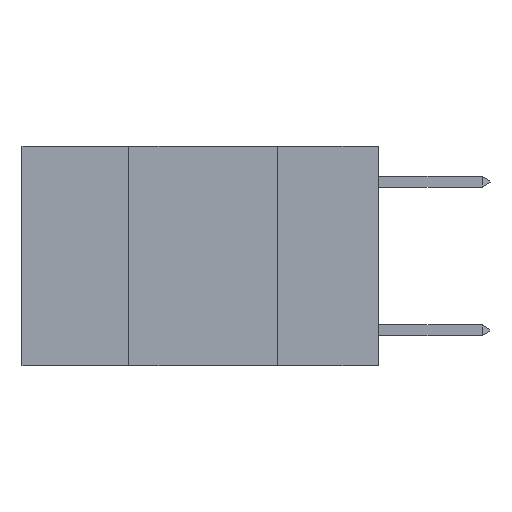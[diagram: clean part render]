
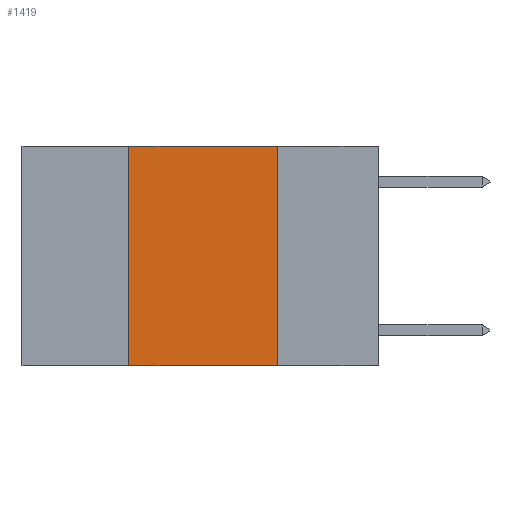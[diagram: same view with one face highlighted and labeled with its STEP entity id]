
A CAD part, left-side view. The second image highlights one B-rep face of the part: STEP entity #1419.
In plain terms, the highlighted planar face has unit normal (-1, 0, 0).
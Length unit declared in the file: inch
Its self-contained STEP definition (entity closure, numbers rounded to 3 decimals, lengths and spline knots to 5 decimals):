
#207 = CARTESIAN_POINT ( 'NONE',  ( 0., 0.17, 0. ) ) ;
#1419 = ADVANCED_FACE ( 'NONE', ( #8242 ), #20766, .F. ) ;
#2036 = VECTOR ( 'NONE', #12750, 39.37008 ) ;
#2325 = DIRECTION ( 'NONE',  ( 0., -1., 0. ) ) ;
#2397 = VERTEX_POINT ( 'NONE', #18102 ) ;
#2954 = LINE ( 'NONE', #10065, #5689 ) ;
#3046 = CARTESIAN_POINT ( 'NONE',  ( 0., 0.42, -0.37 ) ) ;
#3120 = LINE ( 'NONE', #10228, #6499 ) ;
#4056 = LINE ( 'NONE', #207, #2036 ) ;
#5689 = VECTOR ( 'NONE', #17118, 39.37008 ) ;
#6343 = VERTEX_POINT ( 'NONE', #3046 ) ;
#6477 = DIRECTION ( 'NONE',  ( 0., 0., -1. ) ) ;
#6499 = VECTOR ( 'NONE', #12293, 39.37008 ) ;
#6573 = ORIENTED_EDGE ( 'NONE', *, *, #15340, .F. ) ;
#7079 = ORIENTED_EDGE ( 'NONE', *, *, #15444, .F. ) ;
#8242 = FACE_OUTER_BOUND ( 'NONE', #8415, .T. ) ;
#8415 = EDGE_LOOP ( 'NONE', ( #7079, #14793, #6573, #14806 ) ) ;
#10065 = CARTESIAN_POINT ( 'NONE',  ( 0., 0.6, -0.37 ) ) ;
#10228 = CARTESIAN_POINT ( 'NONE',  ( 0., 0.42, 0. ) ) ;
#11942 = CARTESIAN_POINT ( 'NONE',  ( 0., 0.6, 0. ) ) ;
#12293 = DIRECTION ( 'NONE',  ( 0., 0., 1. ) ) ;
#12750 = DIRECTION ( 'NONE',  ( 0., 0., -1. ) ) ;
#14298 = LINE ( 'NONE', #18222, #17286 ) ;
#14793 = ORIENTED_EDGE ( 'NONE', *, *, #22801, .F. ) ;
#14806 = ORIENTED_EDGE ( 'NONE', *, *, #19401, .T. ) ;
#15340 = EDGE_CURVE ( 'NONE', #6343, #15740, #3120, .T. ) ;
#15444 = EDGE_CURVE ( 'NONE', #2397, #16546, #4056, .T. ) ;
#15708 = AXIS2_PLACEMENT_3D ( 'NONE', #11942, #16806, #6477 ) ;
#15740 = VERTEX_POINT ( 'NONE', #22254 ) ;
#16546 = VERTEX_POINT ( 'NONE', #21618 ) ;
#16806 = DIRECTION ( 'NONE',  ( 1., 0., 0. ) ) ;
#17118 = DIRECTION ( 'NONE',  ( 0., -1., 0. ) ) ;
#17286 = VECTOR ( 'NONE', #2325, 39.37008 ) ;
#18102 = CARTESIAN_POINT ( 'NONE',  ( 0., 0.17, 0. ) ) ;
#18222 = CARTESIAN_POINT ( 'NONE',  ( 0., 0.6, 0. ) ) ;
#19401 = EDGE_CURVE ( 'NONE', #6343, #16546, #2954, .T. ) ;
#20766 = PLANE ( 'NONE',  #15708 ) ;
#21618 = CARTESIAN_POINT ( 'NONE',  ( 0., 0.17, -0.37 ) ) ;
#22254 = CARTESIAN_POINT ( 'NONE',  ( 0., 0.42, 0. ) ) ;
#22801 = EDGE_CURVE ( 'NONE', #15740, #2397, #14298, .T. ) ;
